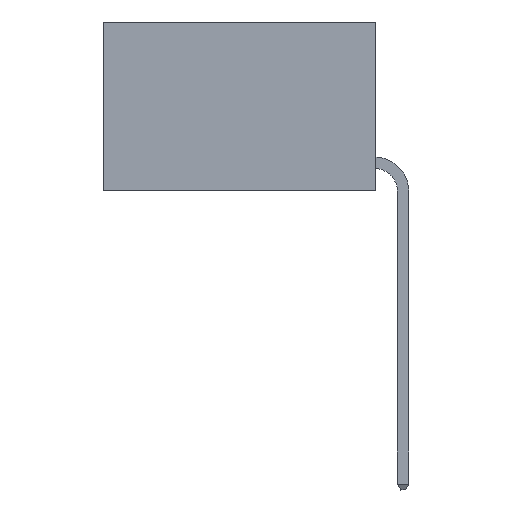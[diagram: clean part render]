
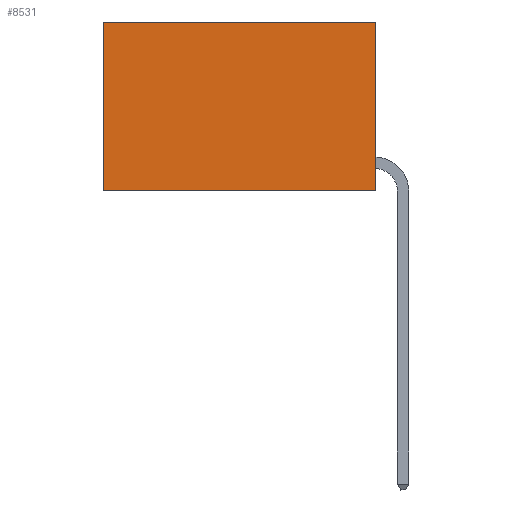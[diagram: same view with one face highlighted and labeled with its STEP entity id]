
A CAD part, left-side view. The second image highlights one B-rep face of the part: STEP entity #8531.
In plain terms, the highlighted planar face has unit normal (-1, 0, 0).
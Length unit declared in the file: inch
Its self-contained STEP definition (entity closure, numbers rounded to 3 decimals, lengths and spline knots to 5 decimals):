
#72 = LINE ( 'NONE', #4101, #248 ) ;
#248 = VECTOR ( 'NONE', #3116, 39.37008 ) ;
#296 = CARTESIAN_POINT ( 'NONE',  ( 0.2625, 0., -0.37 ) ) ;
#526 = DIRECTION ( 'NONE',  ( 0., 1., 0. ) ) ;
#775 = DIRECTION ( 'NONE',  ( 0., 0., -1. ) ) ;
#1522 = DIRECTION ( 'NONE',  ( 0., 1., 0. ) ) ;
#2028 = VERTEX_POINT ( 'NONE', #296 ) ;
#2204 = AXIS2_PLACEMENT_3D ( 'NONE', #5830, #3802, #775 ) ;
#2709 = CARTESIAN_POINT ( 'NONE',  ( 0.2625, 0.6, -0.37 ) ) ;
#3004 = FACE_OUTER_BOUND ( 'NONE', #8967, .T. ) ;
#3116 = DIRECTION ( 'NONE',  ( 0., 0., -1. ) ) ;
#3127 = CARTESIAN_POINT ( 'NONE',  ( 0.2625, 0., 0. ) ) ;
#3416 = VERTEX_POINT ( 'NONE', #3127 ) ;
#3553 = LINE ( 'NONE', #10472, #12229 ) ;
#3802 = DIRECTION ( 'NONE',  ( 1., 0., 0. ) ) ;
#4095 = LINE ( 'NONE', #6747, #6682 ) ;
#4101 = CARTESIAN_POINT ( 'NONE',  ( 0.2625, 0.6, 0. ) ) ;
#4506 = LINE ( 'NONE', #10676, #8798 ) ;
#4535 = VERTEX_POINT ( 'NONE', #6437 ) ;
#5159 = EDGE_CURVE ( 'NONE', #3416, #2028, #4095, .T. ) ;
#5830 = CARTESIAN_POINT ( 'NONE',  ( 0.2625, 0., 0. ) ) ;
#6437 = CARTESIAN_POINT ( 'NONE',  ( 0.2625, 0.6, 0. ) ) ;
#6682 = VECTOR ( 'NONE', #8899, 39.37008 ) ;
#6747 = CARTESIAN_POINT ( 'NONE',  ( 0.2625, 0., 0. ) ) ;
#7060 = PLANE ( 'NONE',  #2204 ) ;
#7442 = ORIENTED_EDGE ( 'NONE', *, *, #9016, .T. ) ;
#7663 = EDGE_CURVE ( 'NONE', #4535, #9545, #72, .T. ) ;
#7950 = EDGE_CURVE ( 'NONE', #2028, #9545, #3553, .T. ) ;
#8149 = ORIENTED_EDGE ( 'NONE', *, *, #5159, .F. ) ;
#8531 = ADVANCED_FACE ( 'NONE', ( #3004 ), #7060, .F. ) ;
#8647 = ORIENTED_EDGE ( 'NONE', *, *, #7950, .F. ) ;
#8798 = VECTOR ( 'NONE', #1522, 39.37008 ) ;
#8899 = DIRECTION ( 'NONE',  ( 0., 0., -1. ) ) ;
#8967 = EDGE_LOOP ( 'NONE', ( #9058, #8647, #8149, #7442 ) ) ;
#9016 = EDGE_CURVE ( 'NONE', #3416, #4535, #4506, .T. ) ;
#9058 = ORIENTED_EDGE ( 'NONE', *, *, #7663, .T. ) ;
#9545 = VERTEX_POINT ( 'NONE', #2709 ) ;
#10472 = CARTESIAN_POINT ( 'NONE',  ( 0.2625, 0., -0.37 ) ) ;
#10676 = CARTESIAN_POINT ( 'NONE',  ( 0.2625, 0., 0. ) ) ;
#12229 = VECTOR ( 'NONE', #526, 39.37008 ) ;
